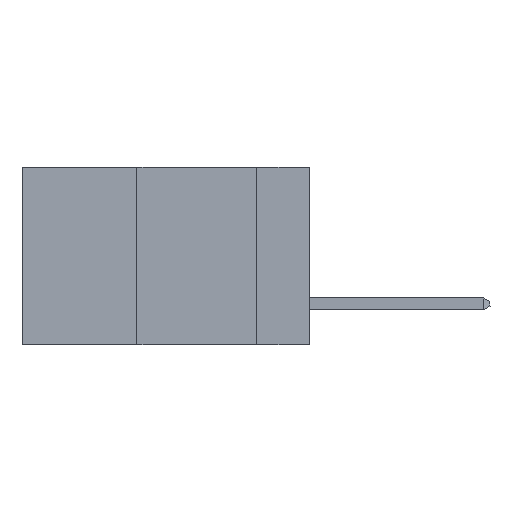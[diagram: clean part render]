
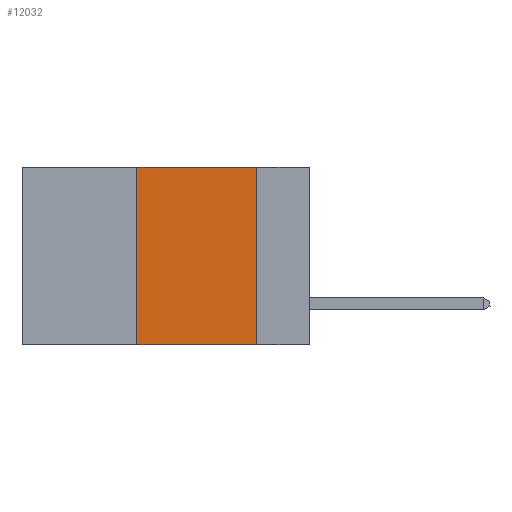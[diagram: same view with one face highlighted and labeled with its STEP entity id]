
A CAD part, left-side view. The second image highlights one B-rep face of the part: STEP entity #12032.
In plain terms, the highlighted planar face has unit normal (-1, 0, 0).
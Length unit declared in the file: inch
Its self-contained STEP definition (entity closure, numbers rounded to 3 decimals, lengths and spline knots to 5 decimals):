
#240 = LINE ( 'NONE', #6615, #752 ) ;
#577 = ORIENTED_EDGE ( 'NONE', *, *, #17724, .F. ) ;
#752 = VECTOR ( 'NONE', #17221, 39.37008 ) ;
#1013 = CARTESIAN_POINT ( 'NONE',  ( 0., 0.11, -0.37 ) ) ;
#1355 = PLANE ( 'NONE',  #6874 ) ;
#2172 = VERTEX_POINT ( 'NONE', #2202 ) ;
#2202 = CARTESIAN_POINT ( 'NONE',  ( 0., 0.36, 0. ) ) ;
#3413 = EDGE_LOOP ( 'NONE', ( #577, #7528, #13474, #13854 ) ) ;
#4810 = VECTOR ( 'NONE', #14667, 39.37008 ) ;
#5858 = LINE ( 'NONE', #7050, #4810 ) ;
#6238 = DIRECTION ( 'NONE',  ( 0., 0., 1. ) ) ;
#6615 = CARTESIAN_POINT ( 'NONE',  ( 0., 0.6, -0.37 ) ) ;
#6874 = AXIS2_PLACEMENT_3D ( 'NONE', #13980, #18397, #9435 ) ;
#7050 = CARTESIAN_POINT ( 'NONE',  ( 0., 0.11, 0. ) ) ;
#7117 = VECTOR ( 'NONE', #6238, 39.37008 ) ;
#7528 = ORIENTED_EDGE ( 'NONE', *, *, #19600, .F. ) ;
#9435 = DIRECTION ( 'NONE',  ( 0., 0., -1. ) ) ;
#9688 = FACE_OUTER_BOUND ( 'NONE', #3413, .T. ) ;
#10189 = VERTEX_POINT ( 'NONE', #15815 ) ;
#10540 = VERTEX_POINT ( 'NONE', #1013 ) ;
#11262 = LINE ( 'NONE', #13504, #14745 ) ;
#12032 = ADVANCED_FACE ( 'NONE', ( #9688 ), #1355, .F. ) ;
#13474 = ORIENTED_EDGE ( 'NONE', *, *, #19197, .F. ) ;
#13504 = CARTESIAN_POINT ( 'NONE',  ( 0., 0.6, 0. ) ) ;
#13648 = VERTEX_POINT ( 'NONE', #19592 ) ;
#13854 = ORIENTED_EDGE ( 'NONE', *, *, #15270, .T. ) ;
#13980 = CARTESIAN_POINT ( 'NONE',  ( 0., 0.6, 0. ) ) ;
#14667 = DIRECTION ( 'NONE',  ( 0., 0., -1. ) ) ;
#14745 = VECTOR ( 'NONE', #19317, 39.37008 ) ;
#15207 = LINE ( 'NONE', #18332, #7117 ) ;
#15270 = EDGE_CURVE ( 'NONE', #10189, #10540, #240, .T. ) ;
#15815 = CARTESIAN_POINT ( 'NONE',  ( 0., 0.36, -0.37 ) ) ;
#17221 = DIRECTION ( 'NONE',  ( 0., -1., 0. ) ) ;
#17724 = EDGE_CURVE ( 'NONE', #13648, #10540, #5858, .T. ) ;
#18332 = CARTESIAN_POINT ( 'NONE',  ( 0., 0.36, 0. ) ) ;
#18397 = DIRECTION ( 'NONE',  ( 1., 0., 0. ) ) ;
#19197 = EDGE_CURVE ( 'NONE', #10189, #2172, #15207, .T. ) ;
#19317 = DIRECTION ( 'NONE',  ( 0., -1., 0. ) ) ;
#19592 = CARTESIAN_POINT ( 'NONE',  ( 0., 0.11, 0. ) ) ;
#19600 = EDGE_CURVE ( 'NONE', #2172, #13648, #11262, .T. ) ;
